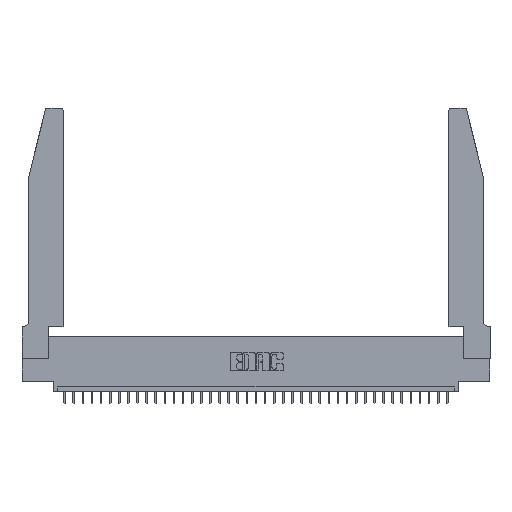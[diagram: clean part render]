
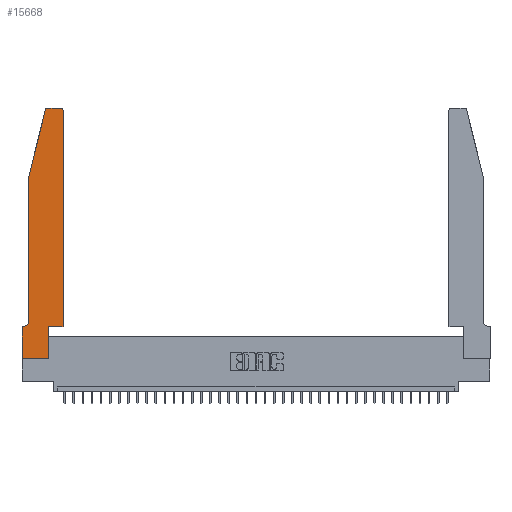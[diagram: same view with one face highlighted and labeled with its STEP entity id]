
A CAD part, top view. The second image highlights one B-rep face of the part: STEP entity #15668.
In plain terms, the highlighted planar face has unit normal (0, 0, 1).
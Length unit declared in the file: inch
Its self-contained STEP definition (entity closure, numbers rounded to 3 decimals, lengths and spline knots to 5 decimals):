
#748 = CARTESIAN_POINT ( 'NONE',  ( 0.284, 2.72, 0.37 ) ) ;
#1038 = PLANE ( 'NONE',  #19350 ) ;
#1282 = VECTOR ( 'NONE', #30643, 39.37008 ) ;
#1343 = CIRCLE ( 'NONE', #35606, 0.03 ) ;
#1492 = CARTESIAN_POINT ( 'NONE',  ( 0.4505, 0.35, 0.37 ) ) ;
#2095 = CARTESIAN_POINT ( 'NONE',  ( 0., 0.35, 0.37 ) ) ;
#2230 = CARTESIAN_POINT ( 'NONE',  ( 0., 0., 0.37 ) ) ;
#2977 = CIRCLE ( 'NONE', #31841, 0.07 ) ;
#3093 = CARTESIAN_POINT ( 'NONE',  ( 0.4505, 0.35, 0.37 ) ) ;
#3426 = EDGE_CURVE ( 'NONE', #21799, #7019, #32608, .T. ) ;
#4091 = DIRECTION ( 'NONE',  ( 0., 0., -1. ) ) ;
#4108 = DIRECTION ( 'NONE',  ( 0., 0., 1. ) ) ;
#4124 = LINE ( 'NONE', #35039, #5539 ) ;
#4253 = VECTOR ( 'NONE', #13493, 39.37008 ) ;
#4802 = CARTESIAN_POINT ( 'NONE',  ( 0.2865, 0.35, 0.37 ) ) ;
#5256 = CARTESIAN_POINT ( 'NONE',  ( 0.2865, 0.35, 0.37 ) ) ;
#5267 = ORIENTED_EDGE ( 'NONE', *, *, #13689, .T. ) ;
#5539 = VECTOR ( 'NONE', #35391, 39.37008 ) ;
#5640 = EDGE_CURVE ( 'NONE', #17336, #9580, #4124, .T. ) ;
#5819 = EDGE_CURVE ( 'NONE', #8225, #13292, #13562, .T. ) ;
#5998 = DIRECTION ( 'NONE',  ( 1., 0., 0. ) ) ;
#6517 = ORIENTED_EDGE ( 'NONE', *, *, #5640, .T. ) ;
#6826 = CARTESIAN_POINT ( 'NONE',  ( 0.0755, 2., 0.37 ) ) ;
#6933 = DIRECTION ( 'NONE',  ( -1., 0., 0. ) ) ;
#7019 = VERTEX_POINT ( 'NONE', #24835 ) ;
#7043 = LINE ( 'NONE', #7222, #15428 ) ;
#7180 = CARTESIAN_POINT ( 'NONE',  ( 0.0755, 2., 0.37 ) ) ;
#7222 = CARTESIAN_POINT ( 'NONE',  ( 0.0755, 0.35, 0.37 ) ) ;
#7852 = VERTEX_POINT ( 'NONE', #15734 ) ;
#7884 = DIRECTION ( 'NONE',  ( 0., -1., 0. ) ) ;
#8225 = VERTEX_POINT ( 'NONE', #14604 ) ;
#9580 = VERTEX_POINT ( 'NONE', #25063 ) ;
#10824 = ORIENTED_EDGE ( 'NONE', *, *, #30754, .T. ) ;
#10967 = VECTOR ( 'NONE', #18314, 39.37008 ) ;
#11109 = LINE ( 'NONE', #2230, #18030 ) ;
#11247 = EDGE_CURVE ( 'NONE', #13292, #35993, #25590, .T. ) ;
#11501 = EDGE_CURVE ( 'NONE', #7019, #18685, #2977, .T. ) ;
#12490 = CARTESIAN_POINT ( 'NONE',  ( 0.0755, 2., 0.37 ) ) ;
#12493 = CARTESIAN_POINT ( 'NONE',  ( 0.25487, 2.72718, 0.37 ) ) ;
#12815 = DIRECTION ( 'NONE',  ( 1., 0., 0. ) ) ;
#13292 = VERTEX_POINT ( 'NONE', #30217 ) ;
#13493 = DIRECTION ( 'NONE',  ( -1., 0., 0. ) ) ;
#13562 = LINE ( 'NONE', #16562, #14629 ) ;
#13642 = EDGE_CURVE ( 'NONE', #35993, #17336, #27062, .T. ) ;
#13689 = EDGE_CURVE ( 'NONE', #23912, #8225, #11109, .T. ) ;
#13819 = VECTOR ( 'NONE', #12815, 39.37008 ) ;
#13855 = ORIENTED_EDGE ( 'NONE', *, *, #3426, .T. ) ;
#14604 = CARTESIAN_POINT ( 'NONE',  ( 0., 0., 0.37 ) ) ;
#14629 = VECTOR ( 'NONE', #27450, 39.37008 ) ;
#14838 = VERTEX_POINT ( 'NONE', #24071 ) ;
#14884 = CARTESIAN_POINT ( 'NONE',  ( 0.4205, 2.72, 0.37 ) ) ;
#15428 = VECTOR ( 'NONE', #35838, 39.37008 ) ;
#15459 = ORIENTED_EDGE ( 'NONE', *, *, #11501, .T. ) ;
#15668 = ADVANCED_FACE ( 'NONE', ( #26799 ), #1038, .T. ) ;
#15734 = CARTESIAN_POINT ( 'NONE',  ( 0.4205, 2.75, 0.37 ) ) ;
#16327 = ORIENTED_EDGE ( 'NONE', *, *, #23200, .T. ) ;
#16562 = CARTESIAN_POINT ( 'NONE',  ( 0., 0., 0.37 ) ) ;
#17336 = VERTEX_POINT ( 'NONE', #3093 ) ;
#17988 = CARTESIAN_POINT ( 'NONE',  ( 0., 0.35, 0.37 ) ) ;
#18030 = VECTOR ( 'NONE', #7884, 39.37008 ) ;
#18314 = DIRECTION ( 'NONE',  ( 0., -1., 0. ) ) ;
#18685 = VERTEX_POINT ( 'NONE', #33005 ) ;
#19326 = AXIS2_PLACEMENT_3D ( 'NONE', #748, #4108, #35748 ) ;
#19350 = AXIS2_PLACEMENT_3D ( 'NONE', #17988, #21366, #30196 ) ;
#20308 = ORIENTED_EDGE ( 'NONE', *, *, #5819, .T. ) ;
#21366 = DIRECTION ( 'NONE',  ( 0., 0., 1. ) ) ;
#21799 = VERTEX_POINT ( 'NONE', #12490 ) ;
#23200 = EDGE_CURVE ( 'NONE', #18685, #23912, #7043, .T. ) ;
#23912 = VERTEX_POINT ( 'NONE', #2095 ) ;
#24071 = CARTESIAN_POINT ( 'NONE',  ( 0.284, 2.75, 0.37 ) ) ;
#24835 = CARTESIAN_POINT ( 'NONE',  ( 0.0755, 0.42, 0.37 ) ) ;
#24839 = DIRECTION ( 'NONE',  ( 0., 1., 0. ) ) ;
#25063 = CARTESIAN_POINT ( 'NONE',  ( 0.4505, 2.72, 0.37 ) ) ;
#25590 = LINE ( 'NONE', #5256, #25819 ) ;
#25819 = VECTOR ( 'NONE', #24839, 39.37008 ) ;
#26175 = VERTEX_POINT ( 'NONE', #12493 ) ;
#26640 = ORIENTED_EDGE ( 'NONE', *, *, #32881, .T. ) ;
#26799 = FACE_OUTER_BOUND ( 'NONE', #27372, .T. ) ;
#27062 = LINE ( 'NONE', #1492, #13819 ) ;
#27372 = EDGE_LOOP ( 'NONE', ( #10824, #36073, #26640, #13855, #15459, #16327, #5267, #20308, #35720, #33930, #6517, #35061 ) ) ;
#27450 = DIRECTION ( 'NONE',  ( 1., 0., 0. ) ) ;
#29528 = DIRECTION ( 'NONE',  ( 0., 0., 1. ) ) ;
#30196 = DIRECTION ( 'NONE',  ( 1., 0., 0. ) ) ;
#30217 = CARTESIAN_POINT ( 'NONE',  ( 0.2865, 0., 0.37 ) ) ;
#30643 = DIRECTION ( 'NONE',  ( -0.239, -0.971, 0. ) ) ;
#30754 = EDGE_CURVE ( 'NONE', #7852, #14838, #33243, .T. ) ;
#30759 = CIRCLE ( 'NONE', #19326, 0.03 ) ;
#31543 = EDGE_CURVE ( 'NONE', #14838, #26175, #30759, .T. ) ;
#31841 = AXIS2_PLACEMENT_3D ( 'NONE', #32723, #4091, #6933 ) ;
#32608 = LINE ( 'NONE', #6826, #10967 ) ;
#32723 = CARTESIAN_POINT ( 'NONE',  ( 0.0055, 0.42, 0.37 ) ) ;
#32881 = EDGE_CURVE ( 'NONE', #26175, #21799, #36667, .T. ) ;
#33005 = CARTESIAN_POINT ( 'NONE',  ( 0.0055, 0.35, 0.37 ) ) ;
#33243 = LINE ( 'NONE', #35695, #4253 ) ;
#33930 = ORIENTED_EDGE ( 'NONE', *, *, #13642, .T. ) ;
#34135 = EDGE_CURVE ( 'NONE', #9580, #7852, #1343, .T. ) ;
#35039 = CARTESIAN_POINT ( 'NONE',  ( 0.4505, 0.35, 0.37 ) ) ;
#35061 = ORIENTED_EDGE ( 'NONE', *, *, #34135, .T. ) ;
#35391 = DIRECTION ( 'NONE',  ( 0., 1., 0. ) ) ;
#35606 = AXIS2_PLACEMENT_3D ( 'NONE', #14884, #29528, #5998 ) ;
#35695 = CARTESIAN_POINT ( 'NONE',  ( 0.2605, 2.75, 0.37 ) ) ;
#35720 = ORIENTED_EDGE ( 'NONE', *, *, #11247, .T. ) ;
#35748 = DIRECTION ( 'NONE',  ( 1., 0., 0. ) ) ;
#35838 = DIRECTION ( 'NONE',  ( -1., 0., 0. ) ) ;
#35993 = VERTEX_POINT ( 'NONE', #4802 ) ;
#36073 = ORIENTED_EDGE ( 'NONE', *, *, #31543, .T. ) ;
#36667 = LINE ( 'NONE', #7180, #1282 ) ;
